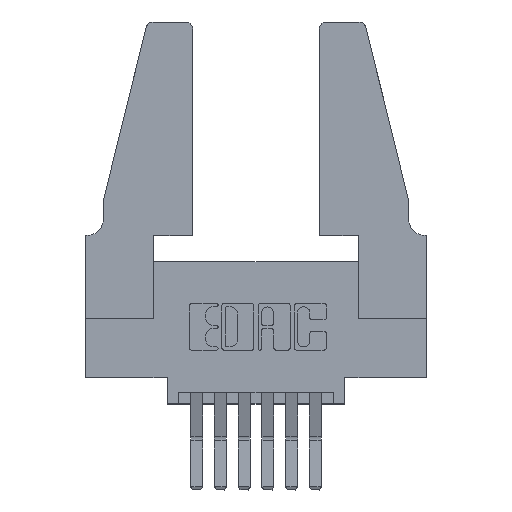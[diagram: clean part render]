
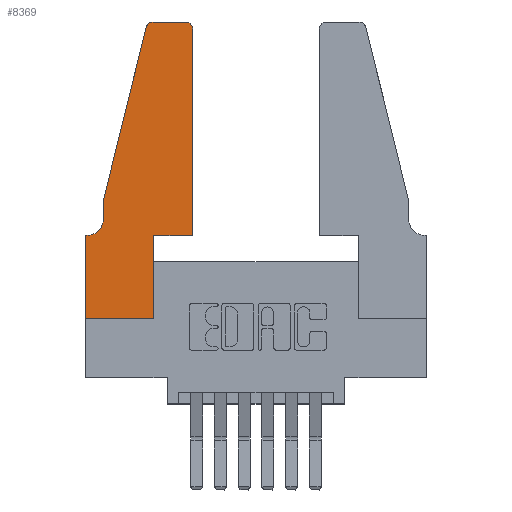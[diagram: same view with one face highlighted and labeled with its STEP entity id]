
A CAD part, top view. The second image highlights one B-rep face of the part: STEP entity #8369.
In plain terms, the highlighted planar face has unit normal (0, 0, 1).
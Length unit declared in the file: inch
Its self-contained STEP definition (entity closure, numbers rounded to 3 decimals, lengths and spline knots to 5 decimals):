
#17 = CARTESIAN_POINT ( 'NONE',  ( 0.4505, 0.35, 0.37 ) ) ;
#19 = AXIS2_PLACEMENT_3D ( 'NONE', #6619, #3848, #7633 ) ;
#87 = EDGE_CURVE ( 'NONE', #11234, #7983, #3319, .T. ) ;
#283 = LINE ( 'NONE', #17, #10382 ) ;
#346 = DIRECTION ( 'NONE',  ( 0., -1., 0. ) ) ;
#391 = VECTOR ( 'NONE', #7781, 39.37008 ) ;
#477 = AXIS2_PLACEMENT_3D ( 'NONE', #2396, #4949, #4816 ) ;
#505 = DIRECTION ( 'NONE',  ( 0., 0., -1. ) ) ;
#545 = VECTOR ( 'NONE', #4005, 39.37008 ) ;
#678 = LINE ( 'NONE', #11914, #10213 ) ;
#1081 = CARTESIAN_POINT ( 'NONE',  ( 0.0055, 0.35, 0.37 ) ) ;
#1153 = DIRECTION ( 'NONE',  ( 0., 0., 1. ) ) ;
#1256 = LINE ( 'NONE', #4165, #391 ) ;
#1306 = LINE ( 'NONE', #10993, #7951 ) ;
#1411 = VERTEX_POINT ( 'NONE', #3145 ) ;
#1460 = VERTEX_POINT ( 'NONE', #4071 ) ;
#1680 = VERTEX_POINT ( 'NONE', #3806 ) ;
#1787 = EDGE_CURVE ( 'NONE', #4296, #10142, #8203, .T. ) ;
#1820 = CARTESIAN_POINT ( 'NONE',  ( 0., 0.35, 0.37 ) ) ;
#1852 = LINE ( 'NONE', #11808, #4437 ) ;
#1941 = CARTESIAN_POINT ( 'NONE',  ( 0.0755, 0.5, 0.37 ) ) ;
#2094 = EDGE_LOOP ( 'NONE', ( #3360, #3356, #9892, #2521, #11409, #2167, #9597, #8885, #5338, #5543, #4773, #8087 ) ) ;
#2126 = AXIS2_PLACEMENT_3D ( 'NONE', #9509, #1153, #3960 ) ;
#2147 = EDGE_CURVE ( 'NONE', #8495, #11234, #2981, .T. ) ;
#2167 = ORIENTED_EDGE ( 'NONE', *, *, #3564, .T. ) ;
#2219 = EDGE_CURVE ( 'NONE', #4310, #3288, #1256, .T. ) ;
#2243 = EDGE_CURVE ( 'NONE', #1680, #4296, #678, .T. ) ;
#2260 = CIRCLE ( 'NONE', #19, 0.03 ) ;
#2396 = CARTESIAN_POINT ( 'NONE',  ( 0., 0.35, 0.37 ) ) ;
#2450 = EDGE_CURVE ( 'NONE', #5262, #1680, #2260, .T. ) ;
#2521 = ORIENTED_EDGE ( 'NONE', *, *, #2147, .T. ) ;
#2781 = DIRECTION ( 'NONE',  ( -1., 0., 0. ) ) ;
#2950 = CARTESIAN_POINT ( 'NONE',  ( 0.0755, 0.5, 0.37 ) ) ;
#2981 = LINE ( 'NONE', #2950, #4570 ) ;
#3145 = CARTESIAN_POINT ( 'NONE',  ( 0.4505, 0.35, 0.37 ) ) ;
#3288 = VERTEX_POINT ( 'NONE', #5782 ) ;
#3319 = CIRCLE ( 'NONE', #11190, 0.07 ) ;
#3356 = ORIENTED_EDGE ( 'NONE', *, *, #1787, .T. ) ;
#3360 = ORIENTED_EDGE ( 'NONE', *, *, #2243, .T. ) ;
#3564 = EDGE_CURVE ( 'NONE', #7983, #11198, #11501, .T. ) ;
#3806 = CARTESIAN_POINT ( 'NONE',  ( 0.4205, 1.25, 0.37 ) ) ;
#3848 = DIRECTION ( 'NONE',  ( 0., 0., 1. ) ) ;
#3960 = DIRECTION ( 'NONE',  ( 1., 0., 0. ) ) ;
#4005 = DIRECTION ( 'NONE',  ( 0., -1., 0. ) ) ;
#4071 = CARTESIAN_POINT ( 'NONE',  ( 0.2865, 0.35, 0.37 ) ) ;
#4119 = VECTOR ( 'NONE', #2781, 39.37008 ) ;
#4165 = CARTESIAN_POINT ( 'NONE',  ( 0., 0., 0.37 ) ) ;
#4296 = VERTEX_POINT ( 'NONE', #7249 ) ;
#4310 = VERTEX_POINT ( 'NONE', #11058 ) ;
#4421 = CARTESIAN_POINT ( 'NONE',  ( 0.0755, 0.35, 0.37 ) ) ;
#4437 = VECTOR ( 'NONE', #7116, 39.37008 ) ;
#4517 = EDGE_CURVE ( 'NONE', #1460, #1411, #4791, .T. ) ;
#4552 = DIRECTION ( 'NONE',  ( -0.239, -0.971, 0. ) ) ;
#4570 = VECTOR ( 'NONE', #346, 39.37008 ) ;
#4636 = VECTOR ( 'NONE', #8822, 39.37008 ) ;
#4773 = ORIENTED_EDGE ( 'NONE', *, *, #7665, .T. ) ;
#4791 = LINE ( 'NONE', #8664, #4636 ) ;
#4816 = DIRECTION ( 'NONE',  ( 1., 0., 0. ) ) ;
#4949 = DIRECTION ( 'NONE',  ( 0., 0., 1. ) ) ;
#5211 = CARTESIAN_POINT ( 'NONE',  ( 0.0055, 0.42, 0.37 ) ) ;
#5262 = VERTEX_POINT ( 'NONE', #10322 ) ;
#5338 = ORIENTED_EDGE ( 'NONE', *, *, #7135, .T. ) ;
#5543 = ORIENTED_EDGE ( 'NONE', *, *, #4517, .T. ) ;
#5782 = CARTESIAN_POINT ( 'NONE',  ( 0.2865, 0., 0.37 ) ) ;
#6288 = EDGE_CURVE ( 'NONE', #10142, #8495, #1306, .T. ) ;
#6508 = DIRECTION ( 'NONE',  ( 0., 1., 0. ) ) ;
#6619 = CARTESIAN_POINT ( 'NONE',  ( 0.4205, 1.22, 0.37 ) ) ;
#7116 = DIRECTION ( 'NONE',  ( 0., 1., 0. ) ) ;
#7135 = EDGE_CURVE ( 'NONE', #3288, #1460, #1852, .T. ) ;
#7237 = PLANE ( 'NONE',  #477 ) ;
#7249 = CARTESIAN_POINT ( 'NONE',  ( 0.284, 1.25, 0.37 ) ) ;
#7633 = DIRECTION ( 'NONE',  ( 1., 0., 0. ) ) ;
#7665 = EDGE_CURVE ( 'NONE', #1411, #5262, #283, .T. ) ;
#7676 = CARTESIAN_POINT ( 'NONE',  ( 0., 0., 0.37 ) ) ;
#7781 = DIRECTION ( 'NONE',  ( 1., 0., 0. ) ) ;
#7951 = VECTOR ( 'NONE', #4552, 39.37008 ) ;
#7983 = VERTEX_POINT ( 'NONE', #1081 ) ;
#8087 = ORIENTED_EDGE ( 'NONE', *, *, #2450, .T. ) ;
#8203 = CIRCLE ( 'NONE', #2126, 0.03 ) ;
#8369 = ADVANCED_FACE ( 'NONE', ( #9640 ), #7237, .T. ) ;
#8495 = VERTEX_POINT ( 'NONE', #1941 ) ;
#8664 = CARTESIAN_POINT ( 'NONE',  ( 0.4505, 0.35, 0.37 ) ) ;
#8822 = DIRECTION ( 'NONE',  ( 1., 0., 0. ) ) ;
#8885 = ORIENTED_EDGE ( 'NONE', *, *, #2219, .T. ) ;
#9341 = CARTESIAN_POINT ( 'NONE',  ( 0.0755, 0.42, 0.37 ) ) ;
#9509 = CARTESIAN_POINT ( 'NONE',  ( 0.284, 1.22, 0.37 ) ) ;
#9597 = ORIENTED_EDGE ( 'NONE', *, *, #10669, .T. ) ;
#9640 = FACE_OUTER_BOUND ( 'NONE', #2094, .T. ) ;
#9676 = DIRECTION ( 'NONE',  ( -1., 0., 0. ) ) ;
#9772 = CARTESIAN_POINT ( 'NONE',  ( 0.25487, 1.22718, 0.37 ) ) ;
#9892 = ORIENTED_EDGE ( 'NONE', *, *, #6288, .T. ) ;
#10142 = VERTEX_POINT ( 'NONE', #9772 ) ;
#10213 = VECTOR ( 'NONE', #11828, 39.37008 ) ;
#10225 = LINE ( 'NONE', #7676, #545 ) ;
#10322 = CARTESIAN_POINT ( 'NONE',  ( 0.4505, 1.22, 0.37 ) ) ;
#10382 = VECTOR ( 'NONE', #6508, 39.37008 ) ;
#10669 = EDGE_CURVE ( 'NONE', #11198, #4310, #10225, .T. ) ;
#10993 = CARTESIAN_POINT ( 'NONE',  ( 0.0755, 0.5, 0.37 ) ) ;
#11058 = CARTESIAN_POINT ( 'NONE',  ( 0., 0., 0.37 ) ) ;
#11190 = AXIS2_PLACEMENT_3D ( 'NONE', #5211, #505, #9676 ) ;
#11198 = VERTEX_POINT ( 'NONE', #1820 ) ;
#11234 = VERTEX_POINT ( 'NONE', #9341 ) ;
#11409 = ORIENTED_EDGE ( 'NONE', *, *, #87, .T. ) ;
#11501 = LINE ( 'NONE', #4421, #4119 ) ;
#11808 = CARTESIAN_POINT ( 'NONE',  ( 0.2865, 0.35, 0.37 ) ) ;
#11828 = DIRECTION ( 'NONE',  ( -1., 0., 0. ) ) ;
#11914 = CARTESIAN_POINT ( 'NONE',  ( 0.2605, 1.25, 0.37 ) ) ;
